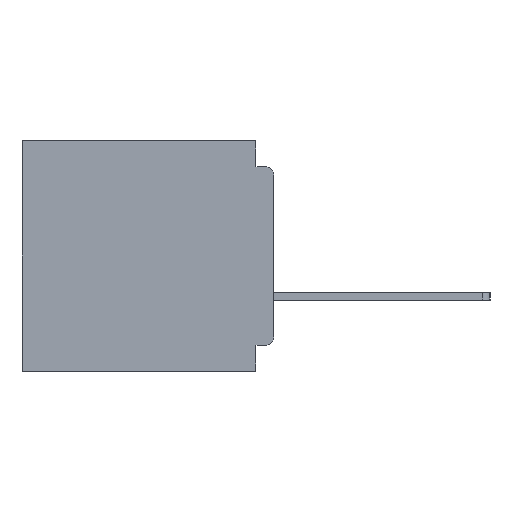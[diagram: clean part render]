
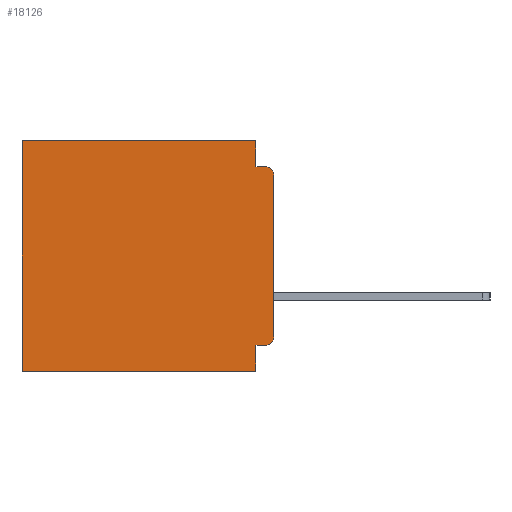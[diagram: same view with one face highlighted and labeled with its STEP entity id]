
A CAD part, left-side view. The second image highlights one B-rep face of the part: STEP entity #18126.
In plain terms, the highlighted planar face has unit normal (-1, 0, 0).
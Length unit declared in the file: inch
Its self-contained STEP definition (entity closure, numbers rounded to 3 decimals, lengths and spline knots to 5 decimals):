
#160 = CARTESIAN_POINT ( 'NONE',  ( 0.3, 0.031, -0.4 ) ) ;
#162 = VERTEX_POINT ( 'NONE', #27137 ) ;
#633 = VECTOR ( 'NONE', #20674, 39.37008 ) ;
#993 = CIRCLE ( 'NONE', #41978, 0.015 ) ;
#1389 = DIRECTION ( 'NONE',  ( 0., 1., 0. ) ) ;
#1725 = ORIENTED_EDGE ( 'NONE', *, *, #31934, .T. ) ;
#1906 = VERTEX_POINT ( 'NONE', #33058 ) ;
#2552 = CARTESIAN_POINT ( 'NONE',  ( 0.3, 0., -0.4 ) ) ;
#3128 = DIRECTION ( 'NONE',  ( 0., 0., -1. ) ) ;
#3413 = EDGE_CURVE ( 'NONE', #1906, #37127, #12932, .T. ) ;
#3482 = EDGE_CURVE ( 'NONE', #27520, #1906, #26325, .T. ) ;
#5094 = CARTESIAN_POINT ( 'NONE',  ( 0.3, 0., -0.4 ) ) ;
#7497 = CARTESIAN_POINT ( 'NONE',  ( 0.3, 0.437, -0.4 ) ) ;
#7682 = EDGE_CURVE ( 'NONE', #18104, #37127, #37479, .T. ) ;
#7866 = LINE ( 'NONE', #36228, #33163 ) ;
#8330 = EDGE_CURVE ( 'NONE', #17997, #162, #10565, .T. ) ;
#8556 = ORIENTED_EDGE ( 'NONE', *, *, #3482, .F. ) ;
#9771 = VECTOR ( 'NONE', #36171, 39.37008 ) ;
#10561 = CARTESIAN_POINT ( 'NONE',  ( 0.3, 0.015, -0.06 ) ) ;
#10565 = LINE ( 'NONE', #7497, #633 ) ;
#11505 = CARTESIAN_POINT ( 'NONE',  ( 0.3, 0.015, -0.34 ) ) ;
#11675 = ORIENTED_EDGE ( 'NONE', *, *, #13785, .F. ) ;
#12932 = LINE ( 'NONE', #41134, #38175 ) ;
#12986 = VECTOR ( 'NONE', #26677, 39.37008 ) ;
#13733 = VERTEX_POINT ( 'NONE', #15689 ) ;
#13757 = ORIENTED_EDGE ( 'NONE', *, *, #32068, .F. ) ;
#13785 = EDGE_CURVE ( 'NONE', #37398, #162, #34475, .T. ) ;
#13939 = DIRECTION ( 'NONE',  ( 0., 0., -1. ) ) ;
#14812 = ORIENTED_EDGE ( 'NONE', *, *, #31737, .F. ) ;
#14853 = DIRECTION ( 'NONE',  ( 0., 0., -1. ) ) ;
#15491 = DIRECTION ( 'NONE',  ( 0., -1., 0. ) ) ;
#15582 = CARTESIAN_POINT ( 'NONE',  ( 0.3, 0.015, -0.355 ) ) ;
#15688 = DIRECTION ( 'NONE',  ( 0., 1., 0. ) ) ;
#15689 = CARTESIAN_POINT ( 'NONE',  ( 0.3, 0.031, -0.355 ) ) ;
#16561 = EDGE_CURVE ( 'NONE', #22945, #38964, #993, .T. ) ;
#17595 = CARTESIAN_POINT ( 'NONE',  ( 0.3, 0.437, 0. ) ) ;
#17997 = VERTEX_POINT ( 'NONE', #17595 ) ;
#18014 = VECTOR ( 'NONE', #25746, 39.37008 ) ;
#18015 = CARTESIAN_POINT ( 'NONE',  ( 0.3, 0., -0.355 ) ) ;
#18104 = VERTEX_POINT ( 'NONE', #41161 ) ;
#18126 = ADVANCED_FACE ( 'NONE', ( #23751 ), #31516, .F. ) ;
#18458 = DIRECTION ( 'NONE',  ( 0., 0., -1. ) ) ;
#18896 = CARTESIAN_POINT ( 'NONE',  ( 0.3, 0.031, 0. ) ) ;
#20674 = DIRECTION ( 'NONE',  ( 0., 0., -1. ) ) ;
#21376 = LINE ( 'NONE', #18015, #29066 ) ;
#21866 = VECTOR ( 'NONE', #15688, 39.37008 ) ;
#22945 = VERTEX_POINT ( 'NONE', #15582 ) ;
#23069 = ORIENTED_EDGE ( 'NONE', *, *, #42722, .F. ) ;
#23406 = CARTESIAN_POINT ( 'NONE',  ( 0.3, 0., -0.4 ) ) ;
#23751 = FACE_OUTER_BOUND ( 'NONE', #24521, .T. ) ;
#24521 = EDGE_LOOP ( 'NONE', ( #23069, #25097, #33855, #8556, #1725, #36932, #11675, #13757, #14812, #38506 ) ) ;
#25097 = ORIENTED_EDGE ( 'NONE', *, *, #7682, .T. ) ;
#25597 = CARTESIAN_POINT ( 'NONE',  ( 0.3, 0., 0. ) ) ;
#25746 = DIRECTION ( 'NONE',  ( 0., 1., 0. ) ) ;
#26325 = LINE ( 'NONE', #38080, #9771 ) ;
#26677 = DIRECTION ( 'NONE',  ( 0., 0., -1. ) ) ;
#27137 = CARTESIAN_POINT ( 'NONE',  ( 0.3, 0.437, -0.4 ) ) ;
#27520 = VERTEX_POINT ( 'NONE', #18896 ) ;
#28467 = CARTESIAN_POINT ( 'NONE',  ( 0.3, 0., -0.34 ) ) ;
#29066 = VECTOR ( 'NONE', #1389, 39.37008 ) ;
#29970 = AXIS2_PLACEMENT_3D ( 'NONE', #10561, #33672, #13939 ) ;
#30477 = LINE ( 'NONE', #23406, #12986 ) ;
#31516 = PLANE ( 'NONE',  #40100 ) ;
#31737 = EDGE_CURVE ( 'NONE', #22945, #13733, #21376, .T. ) ;
#31934 = EDGE_CURVE ( 'NONE', #27520, #17997, #39360, .T. ) ;
#32068 = EDGE_CURVE ( 'NONE', #13733, #37398, #7866, .T. ) ;
#33058 = CARTESIAN_POINT ( 'NONE',  ( 0.3, 0.031, -0.045 ) ) ;
#33163 = VECTOR ( 'NONE', #3128, 39.37008 ) ;
#33672 = DIRECTION ( 'NONE',  ( -1., 0., 0. ) ) ;
#33855 = ORIENTED_EDGE ( 'NONE', *, *, #3413, .F. ) ;
#34475 = LINE ( 'NONE', #2552, #18014 ) ;
#34584 = DIRECTION ( 'NONE',  ( -1., 0., 0. ) ) ;
#36171 = DIRECTION ( 'NONE',  ( 0., 0., -1. ) ) ;
#36228 = CARTESIAN_POINT ( 'NONE',  ( 0.3, 0.031, -0.4 ) ) ;
#36932 = ORIENTED_EDGE ( 'NONE', *, *, #8330, .T. ) ;
#37127 = VERTEX_POINT ( 'NONE', #39770 ) ;
#37398 = VERTEX_POINT ( 'NONE', #160 ) ;
#37479 = CIRCLE ( 'NONE', #29970, 0.015 ) ;
#38080 = CARTESIAN_POINT ( 'NONE',  ( 0.3, 0.031, 0. ) ) ;
#38145 = DIRECTION ( 'NONE',  ( 1., 0., 0. ) ) ;
#38175 = VECTOR ( 'NONE', #15491, 39.37008 ) ;
#38506 = ORIENTED_EDGE ( 'NONE', *, *, #16561, .T. ) ;
#38964 = VERTEX_POINT ( 'NONE', #28467 ) ;
#39360 = LINE ( 'NONE', #25597, #21866 ) ;
#39770 = CARTESIAN_POINT ( 'NONE',  ( 0.3, 0.015, -0.045 ) ) ;
#40100 = AXIS2_PLACEMENT_3D ( 'NONE', #5094, #38145, #18458 ) ;
#41134 = CARTESIAN_POINT ( 'NONE',  ( 0.3, 0., -0.045 ) ) ;
#41161 = CARTESIAN_POINT ( 'NONE',  ( 0.3, 0., -0.06 ) ) ;
#41978 = AXIS2_PLACEMENT_3D ( 'NONE', #11505, #34584, #14853 ) ;
#42722 = EDGE_CURVE ( 'NONE', #18104, #38964, #30477, .T. ) ;
